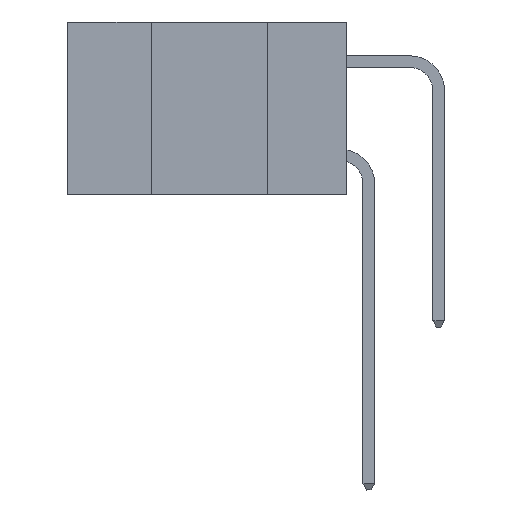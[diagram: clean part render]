
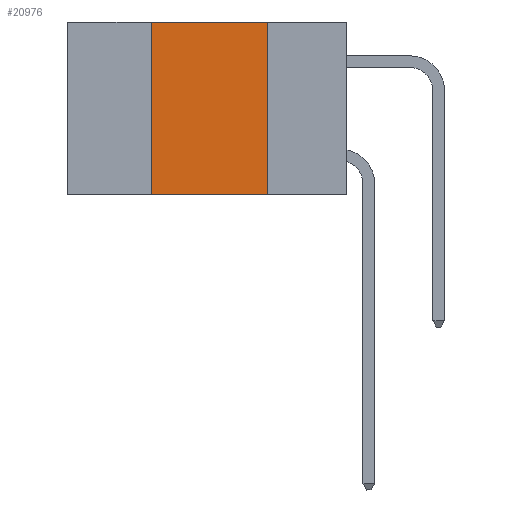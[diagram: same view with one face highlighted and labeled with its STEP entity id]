
A CAD part, left-side view. The second image highlights one B-rep face of the part: STEP entity #20976.
In plain terms, the highlighted planar face has unit normal (-1, 0, 0).
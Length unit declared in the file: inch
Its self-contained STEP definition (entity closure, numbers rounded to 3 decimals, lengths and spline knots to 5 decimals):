
#116 = VERTEX_POINT ( 'NONE', #7543 ) ;
#255 = VERTEX_POINT ( 'NONE', #10530 ) ;
#478 = EDGE_CURVE ( 'NONE', #255, #19142, #19800, .T. ) ;
#507 = DIRECTION ( 'NONE',  ( 0., 0., -1. ) ) ;
#789 = VECTOR ( 'NONE', #9010, 39.37008 ) ;
#2520 = LINE ( 'NONE', #10963, #26341 ) ;
#5167 = VERTEX_POINT ( 'NONE', #22036 ) ;
#5694 = EDGE_CURVE ( 'NONE', #5167, #19142, #19500, .T. ) ;
#5793 = FACE_OUTER_BOUND ( 'NONE', #7062, .T. ) ;
#7062 = EDGE_LOOP ( 'NONE', ( #15694, #23223, #11631, #23738 ) ) ;
#7543 = CARTESIAN_POINT ( 'NONE',  ( 0., 0.42, 0. ) ) ;
#7771 = CARTESIAN_POINT ( 'NONE',  ( 0., 0.17, -0.37 ) ) ;
#8508 = LINE ( 'NONE', #17107, #18190 ) ;
#8551 = DIRECTION ( 'NONE',  ( 1., 0., 0. ) ) ;
#9010 = DIRECTION ( 'NONE',  ( 0., -1., 0. ) ) ;
#9773 = EDGE_CURVE ( 'NONE', #116, #5167, #8508, .T. ) ;
#10530 = CARTESIAN_POINT ( 'NONE',  ( 0., 0.42, -0.37 ) ) ;
#10963 = CARTESIAN_POINT ( 'NONE',  ( 0., 0.42, 0. ) ) ;
#10998 = DIRECTION ( 'NONE',  ( 0., -1., 0. ) ) ;
#11631 = ORIENTED_EDGE ( 'NONE', *, *, #15436, .F. ) ;
#11633 = CARTESIAN_POINT ( 'NONE',  ( 0., 0.6, -0.37 ) ) ;
#15436 = EDGE_CURVE ( 'NONE', #255, #116, #2520, .T. ) ;
#15694 = ORIENTED_EDGE ( 'NONE', *, *, #5694, .F. ) ;
#17107 = CARTESIAN_POINT ( 'NONE',  ( 0., 0.6, 0. ) ) ;
#17202 = DIRECTION ( 'NONE',  ( 0., 0., 1. ) ) ;
#17291 = CARTESIAN_POINT ( 'NONE',  ( 0., 0.17, 0. ) ) ;
#18190 = VECTOR ( 'NONE', #10998, 39.37008 ) ;
#19142 = VERTEX_POINT ( 'NONE', #7771 ) ;
#19500 = LINE ( 'NONE', #17291, #19989 ) ;
#19800 = LINE ( 'NONE', #11633, #789 ) ;
#19989 = VECTOR ( 'NONE', #507, 39.37008 ) ;
#20976 = ADVANCED_FACE ( 'NONE', ( #5793 ), #23115, .F. ) ;
#22036 = CARTESIAN_POINT ( 'NONE',  ( 0., 0.17, 0. ) ) ;
#22043 = AXIS2_PLACEMENT_3D ( 'NONE', #25602, #8551, #22292 ) ;
#22292 = DIRECTION ( 'NONE',  ( 0., 0., -1. ) ) ;
#23115 = PLANE ( 'NONE',  #22043 ) ;
#23223 = ORIENTED_EDGE ( 'NONE', *, *, #9773, .F. ) ;
#23738 = ORIENTED_EDGE ( 'NONE', *, *, #478, .T. ) ;
#25602 = CARTESIAN_POINT ( 'NONE',  ( 0., 0.6, 0. ) ) ;
#26341 = VECTOR ( 'NONE', #17202, 39.37008 ) ;
